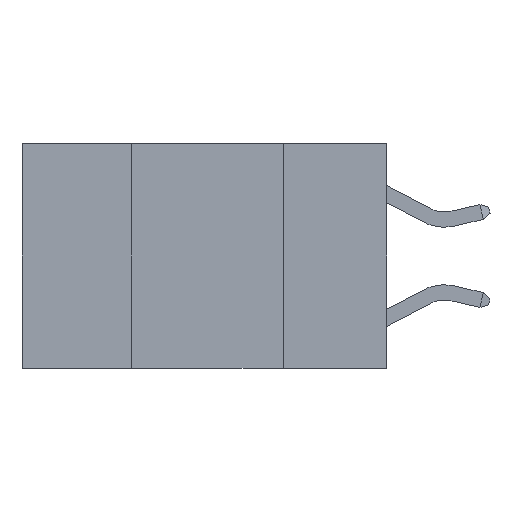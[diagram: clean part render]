
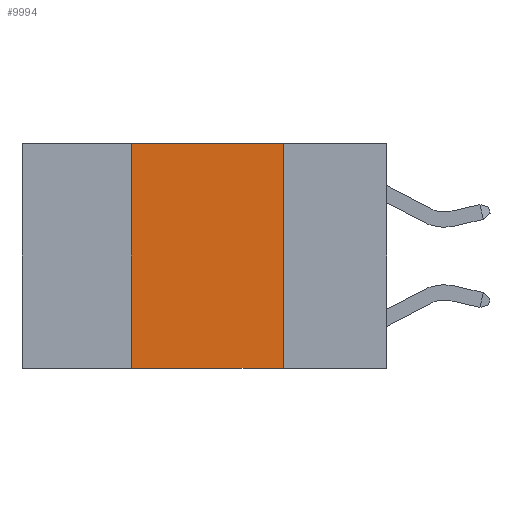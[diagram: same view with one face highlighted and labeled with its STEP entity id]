
A CAD part, left-side view. The second image highlights one B-rep face of the part: STEP entity #9994.
In plain terms, the highlighted planar face has unit normal (-1, 0, 0).
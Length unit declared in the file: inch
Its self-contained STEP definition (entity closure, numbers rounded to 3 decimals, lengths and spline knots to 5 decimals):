
#6 = EDGE_CURVE ( 'NONE', #13107, #2990, #5281, .T. ) ;
#242 = ORIENTED_EDGE ( 'NONE', *, *, #14438, .F. ) ;
#580 = CARTESIAN_POINT ( 'NONE',  ( 0., 0.42, 0. ) ) ;
#666 = ORIENTED_EDGE ( 'NONE', *, *, #6, .T. ) ;
#1896 = EDGE_CURVE ( 'NONE', #8278, #3042, #14640, .T. ) ;
#1915 = CARTESIAN_POINT ( 'NONE',  ( 0., 0.6, 0. ) ) ;
#1938 = DIRECTION ( 'NONE',  ( 0., 0., 1. ) ) ;
#1966 = VECTOR ( 'NONE', #1938, 39.37008 ) ;
#2564 = CARTESIAN_POINT ( 'NONE',  ( 0., 0.6, 0. ) ) ;
#2818 = EDGE_CURVE ( 'NONE', #3042, #2990, #11518, .T. ) ;
#2990 = VERTEX_POINT ( 'NONE', #9237 ) ;
#3042 = VERTEX_POINT ( 'NONE', #8039 ) ;
#3301 = DIRECTION ( 'NONE',  ( 0., 0., -1. ) ) ;
#4030 = FACE_OUTER_BOUND ( 'NONE', #15523, .T. ) ;
#4878 = CARTESIAN_POINT ( 'NONE',  ( 0., 0.17, 0. ) ) ;
#5281 = LINE ( 'NONE', #6343, #11853 ) ;
#5357 = CARTESIAN_POINT ( 'NONE',  ( 0., 0.42, -0.37 ) ) ;
#6182 = AXIS2_PLACEMENT_3D ( 'NONE', #1915, #11214, #3301 ) ;
#6343 = CARTESIAN_POINT ( 'NONE',  ( 0., 0.6, -0.37 ) ) ;
#7908 = DIRECTION ( 'NONE',  ( 0., -1., 0. ) ) ;
#8032 = VECTOR ( 'NONE', #16606, 39.37008 ) ;
#8039 = CARTESIAN_POINT ( 'NONE',  ( 0., 0.17, 0. ) ) ;
#8278 = VERTEX_POINT ( 'NONE', #14231 ) ;
#8555 = PLANE ( 'NONE',  #6182 ) ;
#9051 = LINE ( 'NONE', #580, #1966 ) ;
#9237 = CARTESIAN_POINT ( 'NONE',  ( 0., 0.17, -0.37 ) ) ;
#9994 = ADVANCED_FACE ( 'NONE', ( #4030 ), #8555, .F. ) ;
#10052 = ORIENTED_EDGE ( 'NONE', *, *, #1896, .F. ) ;
#11214 = DIRECTION ( 'NONE',  ( 1., 0., 0. ) ) ;
#11518 = LINE ( 'NONE', #4878, #8032 ) ;
#11853 = VECTOR ( 'NONE', #12974, 39.37008 ) ;
#12974 = DIRECTION ( 'NONE',  ( 0., -1., 0. ) ) ;
#13107 = VERTEX_POINT ( 'NONE', #5357 ) ;
#13137 = ORIENTED_EDGE ( 'NONE', *, *, #2818, .F. ) ;
#14229 = VECTOR ( 'NONE', #7908, 39.37008 ) ;
#14231 = CARTESIAN_POINT ( 'NONE',  ( 0., 0.42, 0. ) ) ;
#14438 = EDGE_CURVE ( 'NONE', #13107, #8278, #9051, .T. ) ;
#14640 = LINE ( 'NONE', #2564, #14229 ) ;
#15523 = EDGE_LOOP ( 'NONE', ( #13137, #10052, #242, #666 ) ) ;
#16606 = DIRECTION ( 'NONE',  ( 0., 0., -1. ) ) ;
